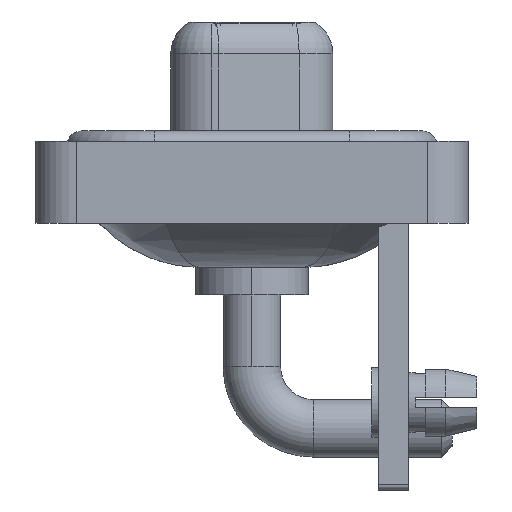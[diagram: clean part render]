
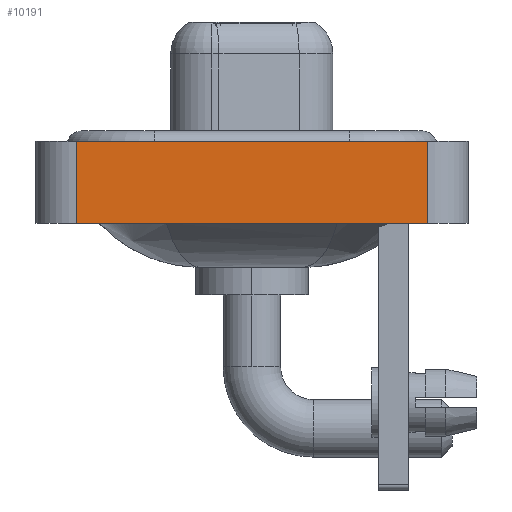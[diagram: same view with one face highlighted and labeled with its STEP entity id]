
A CAD part, left-side view. The second image highlights one B-rep face of the part: STEP entity #10191.
In plain terms, the highlighted planar face has unit normal (-1, 0, 0).
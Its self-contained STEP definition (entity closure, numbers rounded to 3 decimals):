
#161 = LINE ( 'NONE', #13412, #17592 ) ;
#1193 = DIRECTION ( 'NONE',  ( -1., 0., 0. ) ) ;
#1481 = EDGE_CURVE ( 'NONE', #13468, #6892, #5756, .T. ) ;
#1992 = AXIS2_PLACEMENT_3D ( 'NONE', #13901, #1193, #12619 ) ;
#2695 = FACE_OUTER_BOUND ( 'NONE', #17522, .T. ) ;
#3295 = ORIENTED_EDGE ( 'NONE', *, *, #1481, .F. ) ;
#3939 = CARTESIAN_POINT ( 'NONE',  ( -7.3, -8.55, 0.4 ) ) ;
#3984 = CARTESIAN_POINT ( 'NONE',  ( -7.3, 8.55, -3.6 ) ) ;
#4740 = VECTOR ( 'NONE', #16940, 1000. ) ;
#4752 = VECTOR ( 'NONE', #11458, 1000. ) ;
#5537 = VERTEX_POINT ( 'NONE', #10843 ) ;
#5756 = LINE ( 'NONE', #14146, #4752 ) ;
#6446 = LINE ( 'NONE', #16431, #16036 ) ;
#6871 = LINE ( 'NONE', #3984, #4740 ) ;
#6892 = VERTEX_POINT ( 'NONE', #3939 ) ;
#7737 = VERTEX_POINT ( 'NONE', #11083 ) ;
#8110 = DIRECTION ( 'NONE',  ( 0., -1., 0. ) ) ;
#10191 = ADVANCED_FACE ( 'NONE', ( #2695 ), #18190, .T. ) ;
#10476 = ORIENTED_EDGE ( 'NONE', *, *, #13129, .T. ) ;
#10843 = CARTESIAN_POINT ( 'NONE',  ( -7.3, -8.55, -3.6 ) ) ;
#11083 = CARTESIAN_POINT ( 'NONE',  ( -7.3, 8.55, -3.6 ) ) ;
#11458 = DIRECTION ( 'NONE',  ( 0., -1., 0. ) ) ;
#11763 = CARTESIAN_POINT ( 'NONE',  ( -7.3, 8.55, 0.4 ) ) ;
#12027 = DIRECTION ( 'NONE',  ( 0., 0., 1. ) ) ;
#12619 = DIRECTION ( 'NONE',  ( 0., 0., 1. ) ) ;
#12650 = ORIENTED_EDGE ( 'NONE', *, *, #17223, .T. ) ;
#13129 = EDGE_CURVE ( 'NONE', #7737, #5537, #6446, .T. ) ;
#13412 = CARTESIAN_POINT ( 'NONE',  ( -7.3, -8.55, -3.6 ) ) ;
#13468 = VERTEX_POINT ( 'NONE', #11763 ) ;
#13824 = EDGE_CURVE ( 'NONE', #7737, #13468, #6871, .T. ) ;
#13901 = CARTESIAN_POINT ( 'NONE',  ( -7.3, -8.55, -3.6 ) ) ;
#14146 = CARTESIAN_POINT ( 'NONE',  ( -7.3, -8.55, 0.4 ) ) ;
#16036 = VECTOR ( 'NONE', #8110, 1000. ) ;
#16431 = CARTESIAN_POINT ( 'NONE',  ( -7.3, -8.55, -3.6 ) ) ;
#16465 = ORIENTED_EDGE ( 'NONE', *, *, #13824, .F. ) ;
#16940 = DIRECTION ( 'NONE',  ( 0., 0., 1. ) ) ;
#17223 = EDGE_CURVE ( 'NONE', #5537, #6892, #161, .T. ) ;
#17522 = EDGE_LOOP ( 'NONE', ( #12650, #3295, #16465, #10476 ) ) ;
#17592 = VECTOR ( 'NONE', #12027, 1000. ) ;
#18190 = PLANE ( 'NONE',  #1992 ) ;
